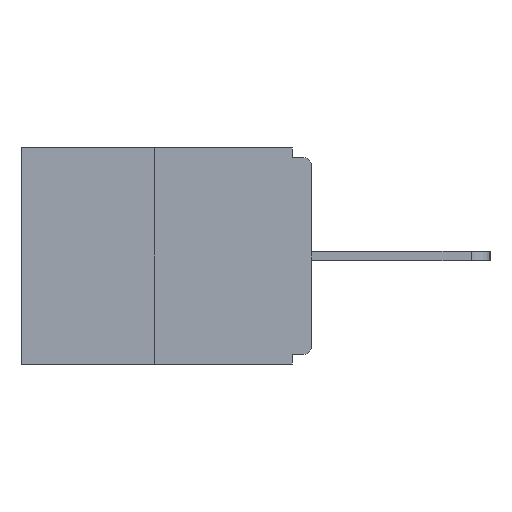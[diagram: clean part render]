
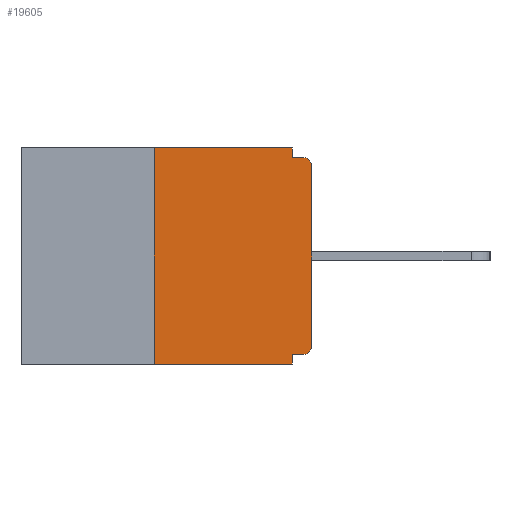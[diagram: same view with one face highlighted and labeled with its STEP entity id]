
A CAD part, left-side view. The second image highlights one B-rep face of the part: STEP entity #19605.
In plain terms, the highlighted planar face has unit normal (-1, 0, 0).
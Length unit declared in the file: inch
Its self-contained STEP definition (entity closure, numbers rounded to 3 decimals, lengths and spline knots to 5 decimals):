
#32 = VERTEX_POINT ( 'NONE', #18836 ) ;
#505 = VECTOR ( 'NONE', #10048, 39.37008 ) ;
#543 = VERTEX_POINT ( 'NONE', #19721 ) ;
#970 = EDGE_CURVE ( 'NONE', #32, #18995, #25472, .T. ) ;
#1101 = ORIENTED_EDGE ( 'NONE', *, *, #8088, .F. ) ;
#1331 = CIRCLE ( 'NONE', #14844, 0.015 ) ;
#1389 = EDGE_CURVE ( 'NONE', #543, #4194, #13442, .T. ) ;
#1667 = CARTESIAN_POINT ( 'NONE',  ( 0., 0., -0.328 ) ) ;
#1851 = VECTOR ( 'NONE', #3989, 39.37008 ) ;
#2310 = EDGE_LOOP ( 'NONE', ( #1101, #11732, #12093, #24749, #2622, #24087, #5427, #18399, #3877, #16780 ) ) ;
#2622 = ORIENTED_EDGE ( 'NONE', *, *, #1389, .F. ) ;
#2787 = CARTESIAN_POINT ( 'NONE',  ( 0., 0.031, -0.015 ) ) ;
#3586 = LINE ( 'NONE', #19035, #505 ) ;
#3604 = LINE ( 'NONE', #22078, #1851 ) ;
#3812 = CARTESIAN_POINT ( 'NONE',  ( 0., 0.015, -0.015 ) ) ;
#3828 = DIRECTION ( 'NONE',  ( 0., 0., -1. ) ) ;
#3877 = ORIENTED_EDGE ( 'NONE', *, *, #4452, .F. ) ;
#3989 = DIRECTION ( 'NONE',  ( 0., 0., 1. ) ) ;
#4194 = VERTEX_POINT ( 'NONE', #16919 ) ;
#4246 = EDGE_CURVE ( 'NONE', #543, #20357, #1331, .T. ) ;
#4452 = EDGE_CURVE ( 'NONE', #6606, #18995, #3586, .T. ) ;
#4900 = DIRECTION ( 'NONE',  ( -1., 0., 0. ) ) ;
#4942 = CARTESIAN_POINT ( 'NONE',  ( 0., 0.46, 0. ) ) ;
#5340 = VECTOR ( 'NONE', #20959, 39.37008 ) ;
#5427 = ORIENTED_EDGE ( 'NONE', *, *, #14003, .T. ) ;
#5498 = CARTESIAN_POINT ( 'NONE',  ( 0., 0., -0.313 ) ) ;
#5678 = LINE ( 'NONE', #13872, #7168 ) ;
#6442 = EDGE_CURVE ( 'NONE', #24921, #17988, #14184, .T. ) ;
#6606 = VERTEX_POINT ( 'NONE', #2787 ) ;
#6616 = DIRECTION ( 'NONE',  ( 0., 0., -1. ) ) ;
#6638 = VERTEX_POINT ( 'NONE', #16535 ) ;
#7168 = VECTOR ( 'NONE', #3828, 39.37008 ) ;
#7956 = DIRECTION ( 'NONE',  ( 0., 0., -1. ) ) ;
#7993 = EDGE_CURVE ( 'NONE', #4194, #6638, #5678, .T. ) ;
#8041 = CARTESIAN_POINT ( 'NONE',  ( 0., 0.031, 0. ) ) ;
#8088 = EDGE_CURVE ( 'NONE', #17988, #23038, #23035, .T. ) ;
#8907 = DIRECTION ( 'NONE',  ( 0., -1., 0. ) ) ;
#10048 = DIRECTION ( 'NONE',  ( 0., -1., 0. ) ) ;
#11732 = ORIENTED_EDGE ( 'NONE', *, *, #6442, .F. ) ;
#12093 = ORIENTED_EDGE ( 'NONE', *, *, #24483, .T. ) ;
#12649 = CARTESIAN_POINT ( 'NONE',  ( 0., 0.46, -0.343 ) ) ;
#13442 = LINE ( 'NONE', #1667, #13501 ) ;
#13501 = VECTOR ( 'NONE', #17533, 39.37008 ) ;
#13650 = PLANE ( 'NONE',  #18893 ) ;
#13872 = CARTESIAN_POINT ( 'NONE',  ( 0., 0.031, -0.343 ) ) ;
#14003 = EDGE_CURVE ( 'NONE', #20357, #32, #3604, .T. ) ;
#14184 = LINE ( 'NONE', #18009, #19142 ) ;
#14534 = AXIS2_PLACEMENT_3D ( 'NONE', #24824, #22474, #6616 ) ;
#14844 = AXIS2_PLACEMENT_3D ( 'NONE', #18166, #4900, #24231 ) ;
#16535 = CARTESIAN_POINT ( 'NONE',  ( 0., 0.031, -0.343 ) ) ;
#16739 = LINE ( 'NONE', #12649, #5340 ) ;
#16780 = ORIENTED_EDGE ( 'NONE', *, *, #22048, .F. ) ;
#16919 = CARTESIAN_POINT ( 'NONE',  ( 0., 0.031, -0.328 ) ) ;
#17533 = DIRECTION ( 'NONE',  ( 0., 1., 0. ) ) ;
#17988 = VERTEX_POINT ( 'NONE', #24690 ) ;
#18009 = CARTESIAN_POINT ( 'NONE',  ( 0., 0.25, 0. ) ) ;
#18166 = CARTESIAN_POINT ( 'NONE',  ( 0., 0.015, -0.313 ) ) ;
#18399 = ORIENTED_EDGE ( 'NONE', *, *, #970, .T. ) ;
#18836 = CARTESIAN_POINT ( 'NONE',  ( 0., 0., -0.03 ) ) ;
#18893 = AXIS2_PLACEMENT_3D ( 'NONE', #19594, #23677, #7956 ) ;
#18995 = VERTEX_POINT ( 'NONE', #3812 ) ;
#19035 = CARTESIAN_POINT ( 'NONE',  ( 0., 0., -0.015 ) ) ;
#19142 = VECTOR ( 'NONE', #24194, 39.37008 ) ;
#19594 = CARTESIAN_POINT ( 'NONE',  ( 0., 0.46, 0. ) ) ;
#19605 = ADVANCED_FACE ( 'NONE', ( #21958 ), #13650, .F. ) ;
#19721 = CARTESIAN_POINT ( 'NONE',  ( 0., 0.015, -0.328 ) ) ;
#20357 = VERTEX_POINT ( 'NONE', #5498 ) ;
#20657 = CARTESIAN_POINT ( 'NONE',  ( 0., 0.031, 0. ) ) ;
#20959 = DIRECTION ( 'NONE',  ( 0., -1., 0. ) ) ;
#21081 = VECTOR ( 'NONE', #8907, 39.37008 ) ;
#21958 = FACE_OUTER_BOUND ( 'NONE', #2310, .T. ) ;
#22048 = EDGE_CURVE ( 'NONE', #23038, #6606, #25857, .T. ) ;
#22078 = CARTESIAN_POINT ( 'NONE',  ( 0., 0., 0. ) ) ;
#22186 = DIRECTION ( 'NONE',  ( 0., 0., -1. ) ) ;
#22474 = DIRECTION ( 'NONE',  ( -1., 0., 0. ) ) ;
#23035 = LINE ( 'NONE', #4942, #21081 ) ;
#23038 = VERTEX_POINT ( 'NONE', #20657 ) ;
#23362 = VECTOR ( 'NONE', #22186, 39.37008 ) ;
#23677 = DIRECTION ( 'NONE',  ( 1., 0., 0. ) ) ;
#24087 = ORIENTED_EDGE ( 'NONE', *, *, #4246, .T. ) ;
#24194 = DIRECTION ( 'NONE',  ( 0., 0., 1. ) ) ;
#24231 = DIRECTION ( 'NONE',  ( 0., 0., -1. ) ) ;
#24483 = EDGE_CURVE ( 'NONE', #24921, #6638, #16739, .T. ) ;
#24690 = CARTESIAN_POINT ( 'NONE',  ( 0., 0.25, 0. ) ) ;
#24749 = ORIENTED_EDGE ( 'NONE', *, *, #7993, .F. ) ;
#24824 = CARTESIAN_POINT ( 'NONE',  ( 0., 0.015, -0.03 ) ) ;
#24921 = VERTEX_POINT ( 'NONE', #25147 ) ;
#25147 = CARTESIAN_POINT ( 'NONE',  ( 0., 0.25, -0.343 ) ) ;
#25472 = CIRCLE ( 'NONE', #14534, 0.015 ) ;
#25857 = LINE ( 'NONE', #8041, #23362 ) ;
